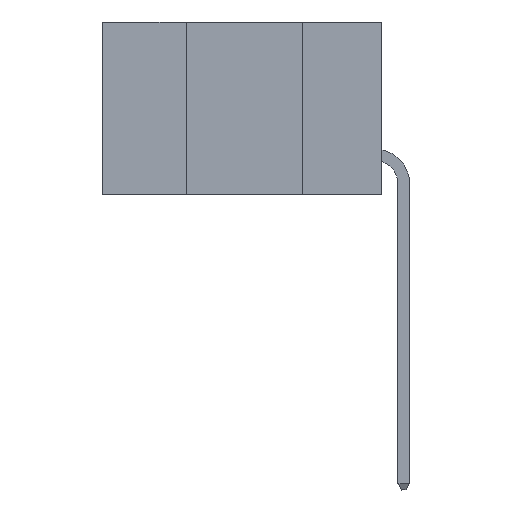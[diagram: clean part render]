
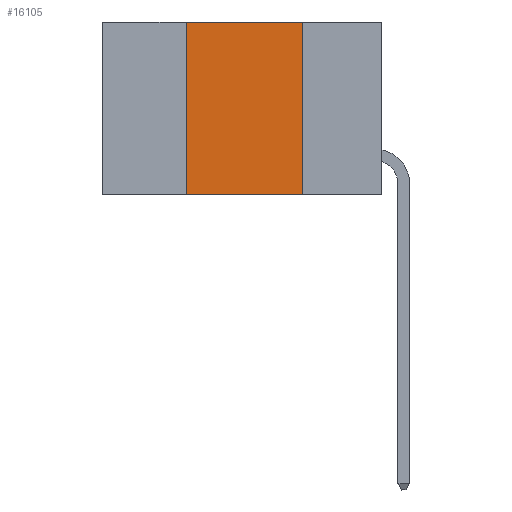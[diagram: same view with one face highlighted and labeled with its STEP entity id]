
A CAD part, left-side view. The second image highlights one B-rep face of the part: STEP entity #16105.
In plain terms, the highlighted planar face has unit normal (-1, 0, 0).
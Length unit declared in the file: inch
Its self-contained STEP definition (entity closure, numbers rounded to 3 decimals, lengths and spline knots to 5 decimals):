
#144 = FACE_OUTER_BOUND ( 'NONE', #2181, .T. ) ;
#266 = CARTESIAN_POINT ( 'NONE',  ( 0., 0.6, 0. ) ) ;
#1462 = VERTEX_POINT ( 'NONE', #3963 ) ;
#1704 = CARTESIAN_POINT ( 'NONE',  ( 0., 0.17, 0. ) ) ;
#1874 = CARTESIAN_POINT ( 'NONE',  ( 0., 0.17, 0. ) ) ;
#2110 = DIRECTION ( 'NONE',  ( 1., 0., 0. ) ) ;
#2181 = EDGE_LOOP ( 'NONE', ( #12623, #14106, #7924, #10627 ) ) ;
#2227 = VECTOR ( 'NONE', #20875, 39.37008 ) ;
#3530 = DIRECTION ( 'NONE',  ( 0., 0., 1. ) ) ;
#3850 = DIRECTION ( 'NONE',  ( 0., 0., -1. ) ) ;
#3963 = CARTESIAN_POINT ( 'NONE',  ( 0., 0.17, -0.37 ) ) ;
#4423 = DIRECTION ( 'NONE',  ( 0., -1., 0. ) ) ;
#5047 = VERTEX_POINT ( 'NONE', #16742 ) ;
#5495 = CARTESIAN_POINT ( 'NONE',  ( 0., 0.42, 0. ) ) ;
#6113 = LINE ( 'NONE', #11583, #19435 ) ;
#6168 = EDGE_CURVE ( 'NONE', #18542, #1462, #6113, .T. ) ;
#7924 = ORIENTED_EDGE ( 'NONE', *, *, #22411, .F. ) ;
#8627 = CARTESIAN_POINT ( 'NONE',  ( 0., 0.6, 0. ) ) ;
#10627 = ORIENTED_EDGE ( 'NONE', *, *, #6168, .T. ) ;
#11507 = LINE ( 'NONE', #1874, #2227 ) ;
#11583 = CARTESIAN_POINT ( 'NONE',  ( 0., 0.6, -0.37 ) ) ;
#12093 = EDGE_CURVE ( 'NONE', #5047, #14263, #21595, .T. ) ;
#12351 = VECTOR ( 'NONE', #16755, 39.37008 ) ;
#12623 = ORIENTED_EDGE ( 'NONE', *, *, #13739, .F. ) ;
#13596 = AXIS2_PLACEMENT_3D ( 'NONE', #266, #2110, #3850 ) ;
#13739 = EDGE_CURVE ( 'NONE', #14263, #1462, #11507, .T. ) ;
#14106 = ORIENTED_EDGE ( 'NONE', *, *, #12093, .F. ) ;
#14263 = VERTEX_POINT ( 'NONE', #1704 ) ;
#14474 = PLANE ( 'NONE',  #13596 ) ;
#16105 = ADVANCED_FACE ( 'NONE', ( #144 ), #14474, .F. ) ;
#16742 = CARTESIAN_POINT ( 'NONE',  ( 0., 0.42, 0. ) ) ;
#16755 = DIRECTION ( 'NONE',  ( 0., -1., 0. ) ) ;
#18542 = VERTEX_POINT ( 'NONE', #22425 ) ;
#19144 = LINE ( 'NONE', #5495, #19669 ) ;
#19435 = VECTOR ( 'NONE', #4423, 39.37008 ) ;
#19669 = VECTOR ( 'NONE', #3530, 39.37008 ) ;
#20875 = DIRECTION ( 'NONE',  ( 0., 0., -1. ) ) ;
#21595 = LINE ( 'NONE', #8627, #12351 ) ;
#22411 = EDGE_CURVE ( 'NONE', #18542, #5047, #19144, .T. ) ;
#22425 = CARTESIAN_POINT ( 'NONE',  ( 0., 0.42, -0.37 ) ) ;
